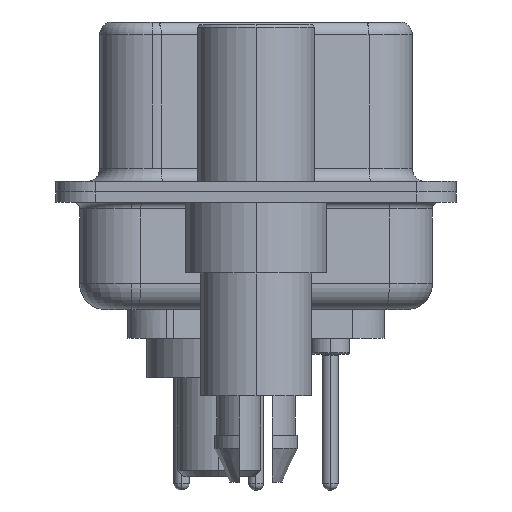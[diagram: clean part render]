
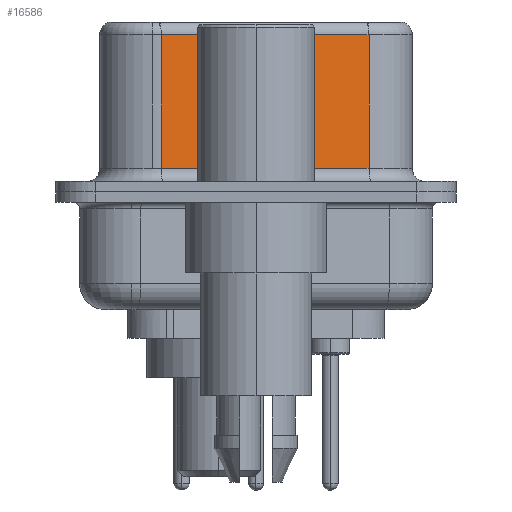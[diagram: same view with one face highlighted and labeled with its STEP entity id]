
A CAD part, left-side view. The second image highlights one B-rep face of the part: STEP entity #16586.
In plain terms, the highlighted planar face has unit normal (-0.985, -0.174, 0).
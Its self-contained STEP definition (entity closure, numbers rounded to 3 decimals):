
#1834 = EDGE_CURVE ( 'NONE', #2907, #14652, #7055, .T. ) ;
#2141 = VECTOR ( 'NONE', #17625, 1000. ) ;
#2721 = FACE_OUTER_BOUND ( 'NONE', #24498, .T. ) ;
#2907 = VERTEX_POINT ( 'NONE', #21148 ) ;
#6385 = VECTOR ( 'NONE', #21329, 1000. ) ;
#7006 = VECTOR ( 'NONE', #25647, 1000. ) ;
#7055 = LINE ( 'NONE', #21407, #6385 ) ;
#7156 = DIRECTION ( 'NONE',  ( 0.174, -0.985, 0. ) ) ;
#8212 = AXIS2_PLACEMENT_3D ( 'NONE', #16706, #8584, #22693 ) ;
#8216 = EDGE_CURVE ( 'NONE', #15200, #2907, #12729, .T. ) ;
#8584 = DIRECTION ( 'NONE',  ( 0.985, 0.174, 0. ) ) ;
#9514 = CARTESIAN_POINT ( 'NONE',  ( 5.132, -4.322, 6.52 ) ) ;
#9784 = CARTESIAN_POINT ( 'NONE',  ( 5.132, -4.322, 0.9 ) ) ;
#10398 = CARTESIAN_POINT ( 'NONE',  ( 5.132, -4.322, 6.02 ) ) ;
#10819 = ORIENTED_EDGE ( 'NONE', *, *, #8216, .T. ) ;
#11364 = CARTESIAN_POINT ( 'NONE',  ( 5.132, -4.322, 0.9 ) ) ;
#12729 = LINE ( 'NONE', #16663, #2141 ) ;
#14408 = ORIENTED_EDGE ( 'NONE', *, *, #1834, .T. ) ;
#14652 = VERTEX_POINT ( 'NONE', #22170 ) ;
#15200 = VERTEX_POINT ( 'NONE', #10398 ) ;
#16586 = ADVANCED_FACE ( 'NONE', ( #2721 ), #16621, .F. ) ;
#16621 = PLANE ( 'NONE',  #8212 ) ;
#16663 = CARTESIAN_POINT ( 'NONE',  ( 5.132, -4.322, 6.02 ) ) ;
#16706 = CARTESIAN_POINT ( 'NONE',  ( 5.132, -4.322, 6.52 ) ) ;
#16963 = VERTEX_POINT ( 'NONE', #9784 ) ;
#17266 = LINE ( 'NONE', #9514, #7006 ) ;
#17625 = DIRECTION ( 'NONE',  ( -0.174, 0.985, 0. ) ) ;
#19579 = VECTOR ( 'NONE', #7156, 1000. ) ;
#21148 = CARTESIAN_POINT ( 'NONE',  ( 3.73, 3.628, 6.02 ) ) ;
#21248 = EDGE_CURVE ( 'NONE', #14652, #16963, #26255, .T. ) ;
#21329 = DIRECTION ( 'NONE',  ( 0., 0., -1. ) ) ;
#21407 = CARTESIAN_POINT ( 'NONE',  ( 3.73, 3.628, 6.52 ) ) ;
#22170 = CARTESIAN_POINT ( 'NONE',  ( 3.73, 3.628, 0.9 ) ) ;
#22228 = ORIENTED_EDGE ( 'NONE', *, *, #21248, .T. ) ;
#22693 = DIRECTION ( 'NONE',  ( -0.174, 0.985, 0. ) ) ;
#24116 = EDGE_CURVE ( 'NONE', #15200, #16963, #17266, .T. ) ;
#24498 = EDGE_LOOP ( 'NONE', ( #25664, #10819, #14408, #22228 ) ) ;
#25647 = DIRECTION ( 'NONE',  ( 0., 0., -1. ) ) ;
#25664 = ORIENTED_EDGE ( 'NONE', *, *, #24116, .F. ) ;
#26255 = LINE ( 'NONE', #11364, #19579 ) ;
